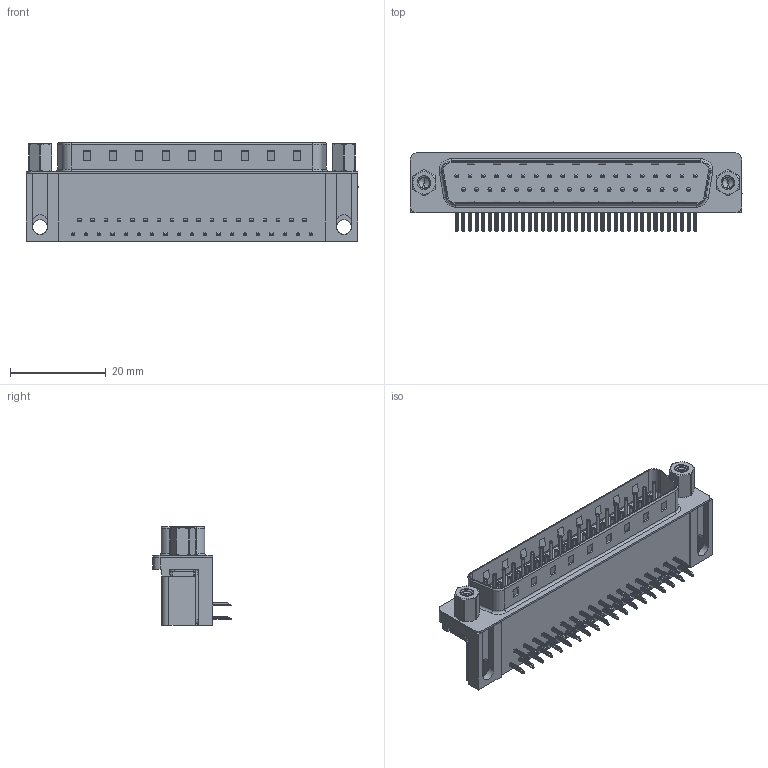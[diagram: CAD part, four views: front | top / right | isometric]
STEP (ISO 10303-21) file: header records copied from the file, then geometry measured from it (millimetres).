
FILE_DESCRIPTION (( 'STEP AP203' ), '1' );
FILE_NAME ('629-037-640-513.STEP', '2021-09-21T21:08:33', ( '' ), ( '' ), 'SwSTEP 2.0', 'SolidWorks 2020', '' );
FILE_SCHEMA (( 'CONFIG_CONTROL_DESIGN' ));
Length unit declared in the file: millimetre
Products named in the file (8): 629 Shell_37 Socket; 629 Contact Top; 629 Contact Bottom; 629-037-640-513; 629 4-40 Threaded Rivet; 629 4-40 Hex Standoff 5; 629 Housing_37 Socket; 629 Thru Hole Board Mount
Assembly tree (45 placements, depth 2):
  629-037-640-513
    629 Housing_37 Socket
    629 Shell_37 Socket
    629 Contact Bottom  x18
    629 Contact Top  x19
    629 Thru Hole Board Mount  x2
    629 4-40 Threaded Rivet  x2
    629 4-40 Hex Standoff 5  x2
Bounding box: 69.4 x 16.35 x 20.6 mm (x, y, z)
Volume: 10178 mm3; surface area: 11276.6 mm2
Topology: 45 solids, 45 shells, 3323 faces, 8247 edges, 5095 vertices
Faces by surface type: plane 2033, cylinder 987, torus 253, cone 32, bspline 18
Entity records: 31528 total; most frequent: CARTESIAN_POINT 9065, DIRECTION 4275, ORIENTED_EDGE 4234, EDGE_CURVE 2117, LINE 1461, VECTOR 1461, AXIS2_PLACEMENT_3D 1407, VERTEX_POINT 1366
